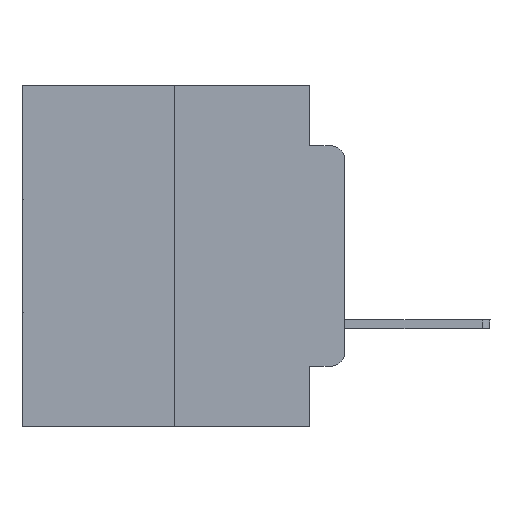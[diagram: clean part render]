
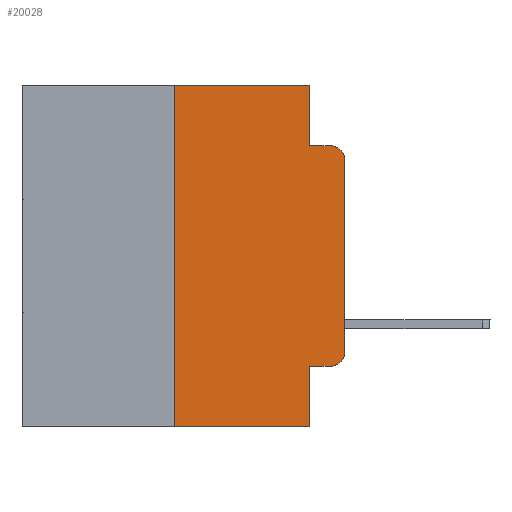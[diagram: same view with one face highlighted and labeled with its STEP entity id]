
A CAD part, left-side view. The second image highlights one B-rep face of the part: STEP entity #20028.
In plain terms, the highlighted planar face has unit normal (-1, 0, 0).
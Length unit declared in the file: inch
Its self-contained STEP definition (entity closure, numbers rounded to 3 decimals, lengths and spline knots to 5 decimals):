
#366 = CARTESIAN_POINT ( 'NONE',  ( 0., 0.051, -0.0885 ) ) ;
#642 = CARTESIAN_POINT ( 'NONE',  ( 0., 0.051, -0.4115 ) ) ;
#1039 = CIRCLE ( 'NONE', #1484, 0.02 ) ;
#1050 = ORIENTED_EDGE ( 'NONE', *, *, #14546, .T. ) ;
#1484 = AXIS2_PLACEMENT_3D ( 'NONE', #10685, #17222, #21076 ) ;
#1705 = LINE ( 'NONE', #17086, #3367 ) ;
#1733 = VECTOR ( 'NONE', #23131, 39.37008 ) ;
#2321 = VERTEX_POINT ( 'NONE', #10613 ) ;
#2386 = DIRECTION ( 'NONE',  ( 0., -1., 0. ) ) ;
#2430 = ORIENTED_EDGE ( 'NONE', *, *, #4373, .F. ) ;
#2477 = AXIS2_PLACEMENT_3D ( 'NONE', #17297, #6791, #9022 ) ;
#2780 = CARTESIAN_POINT ( 'NONE',  ( 0., 0.051, 0. ) ) ;
#2961 = AXIS2_PLACEMENT_3D ( 'NONE', #14090, #3605, #22533 ) ;
#3367 = VECTOR ( 'NONE', #2386, 39.37008 ) ;
#3596 = VERTEX_POINT ( 'NONE', #5271 ) ;
#3605 = DIRECTION ( 'NONE',  ( 1., 0., 0. ) ) ;
#4005 = EDGE_CURVE ( 'NONE', #22267, #3596, #19528, .T. ) ;
#4373 = EDGE_CURVE ( 'NONE', #20912, #4591, #17884, .T. ) ;
#4591 = VERTEX_POINT ( 'NONE', #13294 ) ;
#5271 = CARTESIAN_POINT ( 'NONE',  ( 0., 0.051, -0.5 ) ) ;
#6496 = LINE ( 'NONE', #24594, #7841 ) ;
#6791 = DIRECTION ( 'NONE',  ( -1., 0., 0. ) ) ;
#6816 = FACE_OUTER_BOUND ( 'NONE', #24867, .T. ) ;
#7000 = VERTEX_POINT ( 'NONE', #24506 ) ;
#7680 = VECTOR ( 'NONE', #17389, 39.37008 ) ;
#7800 = CARTESIAN_POINT ( 'NONE',  ( 0., 0.051, 0. ) ) ;
#7841 = VECTOR ( 'NONE', #16261, 39.37008 ) ;
#7917 = LINE ( 'NONE', #10278, #10214 ) ;
#8261 = DIRECTION ( 'NONE',  ( 0., -1., 0. ) ) ;
#8696 = CARTESIAN_POINT ( 'NONE',  ( 0., 0.051, -0.4115 ) ) ;
#9022 = DIRECTION ( 'NONE',  ( 0., 0., -1. ) ) ;
#10214 = VECTOR ( 'NONE', #18846, 39.37008 ) ;
#10278 = CARTESIAN_POINT ( 'NONE',  ( 0., 0.25, 0. ) ) ;
#10280 = EDGE_CURVE ( 'NONE', #13546, #25422, #7917, .T. ) ;
#10583 = CARTESIAN_POINT ( 'NONE',  ( 0., 0.25, -0.5 ) ) ;
#10613 = CARTESIAN_POINT ( 'NONE',  ( 0., 0.02, -0.4115 ) ) ;
#10685 = CARTESIAN_POINT ( 'NONE',  ( 0., 0.02, -0.1085 ) ) ;
#10897 = CARTESIAN_POINT ( 'NONE',  ( 0., 0., 0. ) ) ;
#11123 = CIRCLE ( 'NONE', #2477, 0.02 ) ;
#11268 = EDGE_CURVE ( 'NONE', #2321, #7000, #11123, .T. ) ;
#12282 = CARTESIAN_POINT ( 'NONE',  ( 0., 0.051, -0.0885 ) ) ;
#13273 = ORIENTED_EDGE ( 'NONE', *, *, #10280, .F. ) ;
#13294 = CARTESIAN_POINT ( 'NONE',  ( 0., 0.02, -0.0885 ) ) ;
#13393 = VERTEX_POINT ( 'NONE', #7800 ) ;
#13546 = VERTEX_POINT ( 'NONE', #10583 ) ;
#13830 = PLANE ( 'NONE',  #2961 ) ;
#14090 = CARTESIAN_POINT ( 'NONE',  ( 0., 0.473, 0. ) ) ;
#14546 = EDGE_CURVE ( 'NONE', #16950, #4591, #1039, .T. ) ;
#14963 = LINE ( 'NONE', #10897, #21887 ) ;
#16123 = DIRECTION ( 'NONE',  ( 0., 0., -1. ) ) ;
#16261 = DIRECTION ( 'NONE',  ( 0., -1., 0. ) ) ;
#16950 = VERTEX_POINT ( 'NONE', #26293 ) ;
#17086 = CARTESIAN_POINT ( 'NONE',  ( 0., 0.473, 0. ) ) ;
#17222 = DIRECTION ( 'NONE',  ( -1., 0., 0. ) ) ;
#17297 = CARTESIAN_POINT ( 'NONE',  ( 0., 0.02, -0.3915 ) ) ;
#17344 = DIRECTION ( 'NONE',  ( 0., 0., 1. ) ) ;
#17389 = DIRECTION ( 'NONE',  ( 0., 0., -1. ) ) ;
#17855 = LINE ( 'NONE', #8696, #1733 ) ;
#17877 = EDGE_CURVE ( 'NONE', #7000, #16950, #14963, .T. ) ;
#17884 = LINE ( 'NONE', #12282, #25689 ) ;
#18183 = EDGE_CURVE ( 'NONE', #13393, #20912, #22202, .T. ) ;
#18543 = ORIENTED_EDGE ( 'NONE', *, *, #17877, .T. ) ;
#18846 = DIRECTION ( 'NONE',  ( 0., 0., 1. ) ) ;
#19281 = ORIENTED_EDGE ( 'NONE', *, *, #23987, .F. ) ;
#19528 = LINE ( 'NONE', #2780, #7680 ) ;
#20028 = ADVANCED_FACE ( 'NONE', ( #6816 ), #13830, .F. ) ;
#20912 = VERTEX_POINT ( 'NONE', #366 ) ;
#21076 = DIRECTION ( 'NONE',  ( 0., 0., -1. ) ) ;
#21407 = ORIENTED_EDGE ( 'NONE', *, *, #18183, .F. ) ;
#21887 = VECTOR ( 'NONE', #17344, 39.37008 ) ;
#22044 = ORIENTED_EDGE ( 'NONE', *, *, #4005, .F. ) ;
#22202 = LINE ( 'NONE', #22297, #23492 ) ;
#22267 = VERTEX_POINT ( 'NONE', #642 ) ;
#22297 = CARTESIAN_POINT ( 'NONE',  ( 0., 0.051, 0. ) ) ;
#22533 = DIRECTION ( 'NONE',  ( 0., 0., -1. ) ) ;
#23131 = DIRECTION ( 'NONE',  ( 0., -1., 0. ) ) ;
#23492 = VECTOR ( 'NONE', #16123, 39.37008 ) ;
#23987 = EDGE_CURVE ( 'NONE', #25422, #13393, #1705, .T. ) ;
#24010 = ORIENTED_EDGE ( 'NONE', *, *, #26721, .T. ) ;
#24506 = CARTESIAN_POINT ( 'NONE',  ( 0., 0., -0.3915 ) ) ;
#24594 = CARTESIAN_POINT ( 'NONE',  ( 0., 0.473, -0.5 ) ) ;
#24867 = EDGE_LOOP ( 'NONE', ( #18543, #1050, #2430, #21407, #19281, #13273, #27170, #22044, #24010, #26797 ) ) ;
#25422 = VERTEX_POINT ( 'NONE', #26751 ) ;
#25689 = VECTOR ( 'NONE', #8261, 39.37008 ) ;
#25928 = EDGE_CURVE ( 'NONE', #13546, #3596, #6496, .T. ) ;
#26293 = CARTESIAN_POINT ( 'NONE',  ( 0., 0., -0.1085 ) ) ;
#26721 = EDGE_CURVE ( 'NONE', #22267, #2321, #17855, .T. ) ;
#26751 = CARTESIAN_POINT ( 'NONE',  ( 0., 0.25, 0. ) ) ;
#26797 = ORIENTED_EDGE ( 'NONE', *, *, #11268, .T. ) ;
#27170 = ORIENTED_EDGE ( 'NONE', *, *, #25928, .T. ) ;
